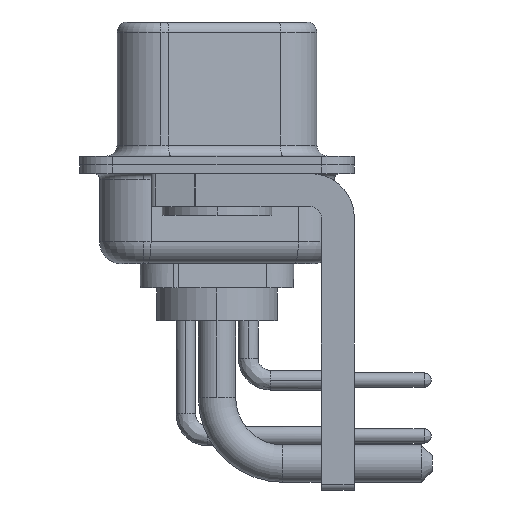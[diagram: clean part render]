
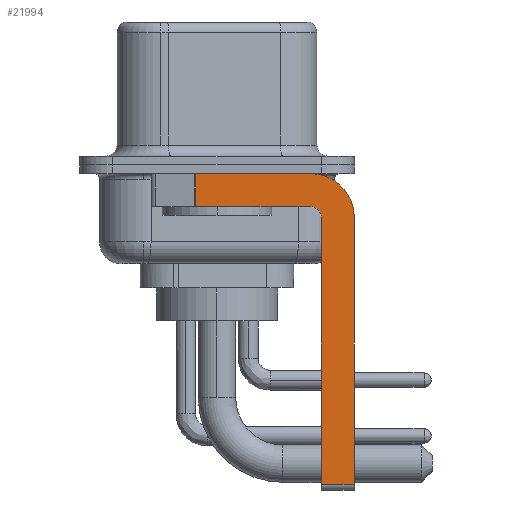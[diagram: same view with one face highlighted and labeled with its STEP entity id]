
A CAD part, left-side view. The second image highlights one B-rep face of the part: STEP entity #21994.
In plain terms, the highlighted planar face has unit normal (-1, 0, 0).
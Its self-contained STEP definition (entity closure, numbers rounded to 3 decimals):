
#649 = VECTOR ( 'NONE', #2091, 1000. ) ;
#795 = CARTESIAN_POINT ( 'NONE',  ( -2.9, 3., -0.4 ) ) ;
#925 = VERTEX_POINT ( 'NONE', #14225 ) ;
#1149 = DIRECTION ( 'NONE',  ( 0., -1., 0. ) ) ;
#2091 = DIRECTION ( 'NONE',  ( 0., -1., 0. ) ) ;
#2524 = DIRECTION ( 'NONE',  ( 0., 0., -1. ) ) ;
#2560 = LINE ( 'NONE', #4203, #649 ) ;
#2633 = VERTEX_POINT ( 'NONE', #7986 ) ;
#3335 = EDGE_CURVE ( 'NONE', #13244, #925, #17895, .T. ) ;
#3781 = CIRCLE ( 'NONE', #13136, 2. ) ;
#4203 = CARTESIAN_POINT ( 'NONE',  ( -2.9, -4.25, -14.55 ) ) ;
#4452 = ORIENTED_EDGE ( 'NONE', *, *, #8726, .F. ) ;
#4633 = FACE_OUTER_BOUND ( 'NONE', #18169, .T. ) ;
#4742 = ORIENTED_EDGE ( 'NONE', *, *, #14941, .F. ) ;
#5357 = DIRECTION ( 'NONE',  ( 0., 0., 1. ) ) ;
#5370 = LINE ( 'NONE', #21557, #23084 ) ;
#5783 = EDGE_CURVE ( 'NONE', #13244, #12863, #2560, .T. ) ;
#6278 = DIRECTION ( 'NONE',  ( 1., 0., 0. ) ) ;
#6292 = DIRECTION ( 'NONE',  ( 0., 0., -1. ) ) ;
#6381 = DIRECTION ( 'NONE',  ( 0., 0., -1. ) ) ;
#6744 = VECTOR ( 'NONE', #6381, 1000. ) ;
#7497 = ORIENTED_EDGE ( 'NONE', *, *, #3335, .F. ) ;
#7602 = VECTOR ( 'NONE', #17361, 1000. ) ;
#7986 = CARTESIAN_POINT ( 'NONE',  ( -2.9, 0.978, -0.4 ) ) ;
#8031 = CARTESIAN_POINT ( 'NONE',  ( -2.9, 0.978, -1.9 ) ) ;
#8257 = CARTESIAN_POINT ( 'NONE',  ( -2.9, -6.25, -2.4 ) ) ;
#8304 = ORIENTED_EDGE ( 'NONE', *, *, #16048, .F. ) ;
#8726 = EDGE_CURVE ( 'NONE', #925, #20639, #11655, .T. ) ;
#8855 = ORIENTED_EDGE ( 'NONE', *, *, #18624, .F. ) ;
#10027 = CARTESIAN_POINT ( 'NONE',  ( -2.9, -4.25, -2.4 ) ) ;
#10219 = CARTESIAN_POINT ( 'NONE',  ( -2.9, 0.978, -1.9 ) ) ;
#10536 = DIRECTION ( 'NONE',  ( 0., 1., 0. ) ) ;
#10921 = CARTESIAN_POINT ( 'NONE',  ( -2.9, -4.25, -2.4 ) ) ;
#11390 = DIRECTION ( 'NONE',  ( -1., 0., 0. ) ) ;
#11655 = CIRCLE ( 'NONE', #13144, 0.5 ) ;
#12607 = ORIENTED_EDGE ( 'NONE', *, *, #18205, .T. ) ;
#12626 = VERTEX_POINT ( 'NONE', #14271 ) ;
#12860 = VECTOR ( 'NONE', #1149, 1000. ) ;
#12863 = VERTEX_POINT ( 'NONE', #16495 ) ;
#13136 = AXIS2_PLACEMENT_3D ( 'NONE', #13555, #22360, #6292 ) ;
#13144 = AXIS2_PLACEMENT_3D ( 'NONE', #10921, #11390, #21816 ) ;
#13182 = CARTESIAN_POINT ( 'NONE',  ( -2.9, -4.25, -1.9 ) ) ;
#13244 = VERTEX_POINT ( 'NONE', #18911 ) ;
#13247 = LINE ( 'NONE', #795, #12860 ) ;
#13321 = AXIS2_PLACEMENT_3D ( 'NONE', #10027, #6278, #2524 ) ;
#13555 = CARTESIAN_POINT ( 'NONE',  ( -2.9, -4.25, -2.4 ) ) ;
#14225 = CARTESIAN_POINT ( 'NONE',  ( -2.9, -4.75, -2.4 ) ) ;
#14271 = CARTESIAN_POINT ( 'NONE',  ( -2.9, -6.25, -2.4 ) ) ;
#14941 = EDGE_CURVE ( 'NONE', #12626, #12863, #22451, .T. ) ;
#16048 = EDGE_CURVE ( 'NONE', #20836, #12626, #3781, .T. ) ;
#16129 = CARTESIAN_POINT ( 'NONE',  ( -2.9, -4.75, -14.8 ) ) ;
#16495 = CARTESIAN_POINT ( 'NONE',  ( -2.9, -6.25, -14.55 ) ) ;
#17361 = DIRECTION ( 'NONE',  ( 0., 0., -1. ) ) ;
#17870 = VERTEX_POINT ( 'NONE', #8031 ) ;
#17895 = LINE ( 'NONE', #16129, #18940 ) ;
#18169 = EDGE_LOOP ( 'NONE', ( #8855, #12607, #21523, #4452, #7497, #22333, #4742, #8304 ) ) ;
#18205 = EDGE_CURVE ( 'NONE', #2633, #17870, #20436, .T. ) ;
#18585 = PLANE ( 'NONE',  #13321 ) ;
#18624 = EDGE_CURVE ( 'NONE', #2633, #20836, #13247, .T. ) ;
#18911 = CARTESIAN_POINT ( 'NONE',  ( -2.9, -4.75, -14.55 ) ) ;
#18940 = VECTOR ( 'NONE', #5357, 1000. ) ;
#20084 = CARTESIAN_POINT ( 'NONE',  ( -2.9, -4.25, -0.4 ) ) ;
#20436 = LINE ( 'NONE', #10219, #7602 ) ;
#20639 = VERTEX_POINT ( 'NONE', #13182 ) ;
#20836 = VERTEX_POINT ( 'NONE', #20084 ) ;
#21523 = ORIENTED_EDGE ( 'NONE', *, *, #22947, .F. ) ;
#21557 = CARTESIAN_POINT ( 'NONE',  ( -2.9, -4.25, -1.9 ) ) ;
#21816 = DIRECTION ( 'NONE',  ( 0., 0., 1. ) ) ;
#21994 = ADVANCED_FACE ( 'NONE', ( #4633 ), #18585, .F. ) ;
#22333 = ORIENTED_EDGE ( 'NONE', *, *, #5783, .T. ) ;
#22360 = DIRECTION ( 'NONE',  ( 1., 0., 0. ) ) ;
#22451 = LINE ( 'NONE', #8257, #6744 ) ;
#22947 = EDGE_CURVE ( 'NONE', #20639, #17870, #5370, .T. ) ;
#23084 = VECTOR ( 'NONE', #10536, 1000. ) ;
